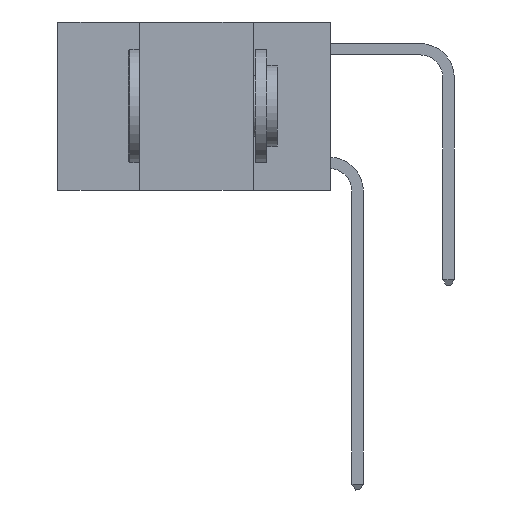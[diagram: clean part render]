
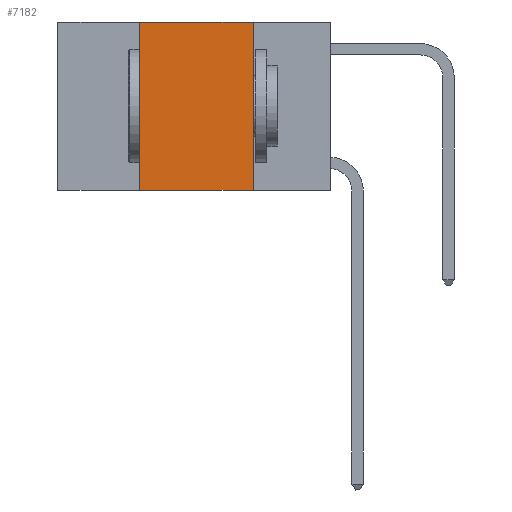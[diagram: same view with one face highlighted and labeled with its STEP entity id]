
A CAD part, left-side view. The second image highlights one B-rep face of the part: STEP entity #7182.
In plain terms, the highlighted planar face has unit normal (-1, 0, 0).
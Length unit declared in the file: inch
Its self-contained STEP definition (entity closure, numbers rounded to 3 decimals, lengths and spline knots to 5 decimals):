
#1069 = EDGE_LOOP ( 'NONE', ( #16432, #15061, #15940, #6046 ) ) ;
#1159 = CARTESIAN_POINT ( 'NONE',  ( 0., 0.42, -0.37 ) ) ;
#1193 = DIRECTION ( 'NONE',  ( 0., -1., 0. ) ) ;
#1401 = EDGE_CURVE ( 'NONE', #8680, #10790, #19468, .T. ) ;
#1966 = VERTEX_POINT ( 'NONE', #14117 ) ;
#1976 = EDGE_CURVE ( 'NONE', #1966, #6648, #3092, .T. ) ;
#2676 = DIRECTION ( 'NONE',  ( 0., 0., -1. ) ) ;
#3092 = LINE ( 'NONE', #16136, #15176 ) ;
#3138 = CARTESIAN_POINT ( 'NONE',  ( 0., 0.17, 0. ) ) ;
#3409 = DIRECTION ( 'NONE',  ( 0., 0., 1. ) ) ;
#3613 = CARTESIAN_POINT ( 'NONE',  ( 0., 0.42, 0. ) ) ;
#3629 = CARTESIAN_POINT ( 'NONE',  ( 0., 0.6, 0. ) ) ;
#3652 = VECTOR ( 'NONE', #2676, 39.37008 ) ;
#3928 = VECTOR ( 'NONE', #1193, 39.37008 ) ;
#6046 = ORIENTED_EDGE ( 'NONE', *, *, #1401, .T. ) ;
#6648 = VERTEX_POINT ( 'NONE', #3138 ) ;
#7182 = ADVANCED_FACE ( 'NONE', ( #13692 ), #18272, .F. ) ;
#8680 = VERTEX_POINT ( 'NONE', #1159 ) ;
#9462 = EDGE_CURVE ( 'NONE', #8680, #1966, #11552, .T. ) ;
#9555 = CARTESIAN_POINT ( 'NONE',  ( 0., 0.17, -0.37 ) ) ;
#10790 = VERTEX_POINT ( 'NONE', #9555 ) ;
#11552 = LINE ( 'NONE', #3613, #19547 ) ;
#13692 = FACE_OUTER_BOUND ( 'NONE', #1069, .T. ) ;
#13784 = DIRECTION ( 'NONE',  ( 1., 0., 0. ) ) ;
#14117 = CARTESIAN_POINT ( 'NONE',  ( 0., 0.42, 0. ) ) ;
#15061 = ORIENTED_EDGE ( 'NONE', *, *, #1976, .F. ) ;
#15176 = VECTOR ( 'NONE', #19856, 39.37008 ) ;
#15180 = DIRECTION ( 'NONE',  ( 0., 0., -1. ) ) ;
#15382 = AXIS2_PLACEMENT_3D ( 'NONE', #3629, #13784, #15180 ) ;
#15833 = CARTESIAN_POINT ( 'NONE',  ( 0., 0.17, 0. ) ) ;
#15895 = EDGE_CURVE ( 'NONE', #6648, #10790, #17433, .T. ) ;
#15940 = ORIENTED_EDGE ( 'NONE', *, *, #9462, .F. ) ;
#16136 = CARTESIAN_POINT ( 'NONE',  ( 0., 0.6, 0. ) ) ;
#16432 = ORIENTED_EDGE ( 'NONE', *, *, #15895, .F. ) ;
#17433 = LINE ( 'NONE', #15833, #3652 ) ;
#18272 = PLANE ( 'NONE',  #15382 ) ;
#19468 = LINE ( 'NONE', #20755, #3928 ) ;
#19547 = VECTOR ( 'NONE', #3409, 39.37008 ) ;
#19856 = DIRECTION ( 'NONE',  ( 0., -1., 0. ) ) ;
#20755 = CARTESIAN_POINT ( 'NONE',  ( 0., 0.6, -0.37 ) ) ;
